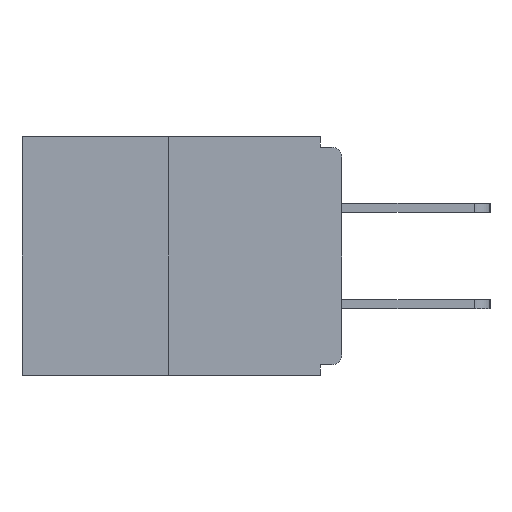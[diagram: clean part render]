
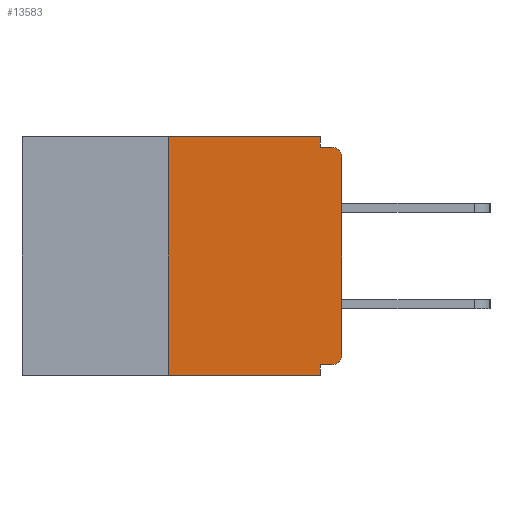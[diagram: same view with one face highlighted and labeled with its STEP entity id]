
A CAD part, left-side view. The second image highlights one B-rep face of the part: STEP entity #13583.
In plain terms, the highlighted planar face has unit normal (-1, 0, 0).
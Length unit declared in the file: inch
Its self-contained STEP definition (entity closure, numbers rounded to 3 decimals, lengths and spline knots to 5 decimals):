
#109 = CARTESIAN_POINT ( 'NONE',  ( 0., 0.031, -0.343 ) ) ;
#119 = ORIENTED_EDGE ( 'NONE', *, *, #7556, .F. ) ;
#203 = VECTOR ( 'NONE', #896, 39.37008 ) ;
#543 = DIRECTION ( 'NONE',  ( 0., -1., 0. ) ) ;
#877 = DIRECTION ( 'NONE',  ( 0., 0., 1. ) ) ;
#896 = DIRECTION ( 'NONE',  ( 0., -1., 0. ) ) ;
#913 = VERTEX_POINT ( 'NONE', #11214 ) ;
#1031 = FACE_OUTER_BOUND ( 'NONE', #7024, .T. ) ;
#1077 = VERTEX_POINT ( 'NONE', #8157 ) ;
#1084 = LINE ( 'NONE', #14793, #8114 ) ;
#1231 = CARTESIAN_POINT ( 'NONE',  ( 0., 0.031, -0.328 ) ) ;
#1260 = VERTEX_POINT ( 'NONE', #14646 ) ;
#1440 = EDGE_CURVE ( 'NONE', #9782, #913, #1084, .T. ) ;
#2194 = EDGE_CURVE ( 'NONE', #5644, #6878, #12732, .T. ) ;
#2239 = CARTESIAN_POINT ( 'NONE',  ( 0., 0.46, 0. ) ) ;
#2251 = ORIENTED_EDGE ( 'NONE', *, *, #5834, .T. ) ;
#2365 = VECTOR ( 'NONE', #12906, 39.37008 ) ;
#2741 = CARTESIAN_POINT ( 'NONE',  ( 0., 0.25, 0. ) ) ;
#2945 = VERTEX_POINT ( 'NONE', #2741 ) ;
#2973 = DIRECTION ( 'NONE',  ( 0., 0., 1. ) ) ;
#3752 = VERTEX_POINT ( 'NONE', #109 ) ;
#3786 = EDGE_CURVE ( 'NONE', #1260, #8052, #11182, .T. ) ;
#3901 = CARTESIAN_POINT ( 'NONE',  ( 0., 0.031, 0. ) ) ;
#3921 = ORIENTED_EDGE ( 'NONE', *, *, #3786, .T. ) ;
#4230 = VECTOR ( 'NONE', #543, 39.37008 ) ;
#4291 = ORIENTED_EDGE ( 'NONE', *, *, #6235, .F. ) ;
#4320 = LINE ( 'NONE', #8643, #4230 ) ;
#4352 = DIRECTION ( 'NONE',  ( 0., 0., -1. ) ) ;
#4830 = ORIENTED_EDGE ( 'NONE', *, *, #2194, .F. ) ;
#4906 = DIRECTION ( 'NONE',  ( 0., 0., -1. ) ) ;
#5644 = VERTEX_POINT ( 'NONE', #11697 ) ;
#5726 = DIRECTION ( 'NONE',  ( 1., 0., 0. ) ) ;
#5761 = CIRCLE ( 'NONE', #14292, 0.015 ) ;
#5834 = EDGE_CURVE ( 'NONE', #6703, #3752, #4320, .T. ) ;
#6095 = DIRECTION ( 'NONE',  ( 0., -1., 0. ) ) ;
#6235 = EDGE_CURVE ( 'NONE', #6703, #2945, #11353, .T. ) ;
#6686 = AXIS2_PLACEMENT_3D ( 'NONE', #11919, #8271, #8411 ) ;
#6703 = VERTEX_POINT ( 'NONE', #11028 ) ;
#6878 = VERTEX_POINT ( 'NONE', #1231 ) ;
#7024 = EDGE_LOOP ( 'NONE', ( #119, #4291, #2251, #10274, #4830, #8607, #3921, #10538, #7695, #13359 ) ) ;
#7244 = VECTOR ( 'NONE', #2973, 39.37008 ) ;
#7411 = CIRCLE ( 'NONE', #6686, 0.015 ) ;
#7556 = EDGE_CURVE ( 'NONE', #2945, #9782, #11292, .T. ) ;
#7694 = CARTESIAN_POINT ( 'NONE',  ( 0., 0.25, 0. ) ) ;
#7695 = ORIENTED_EDGE ( 'NONE', *, *, #10956, .F. ) ;
#7779 = CARTESIAN_POINT ( 'NONE',  ( 0., 0., -0.03 ) ) ;
#7876 = EDGE_CURVE ( 'NONE', #5644, #1260, #5761, .T. ) ;
#8052 = VERTEX_POINT ( 'NONE', #7779 ) ;
#8114 = VECTOR ( 'NONE', #4352, 39.37008 ) ;
#8157 = CARTESIAN_POINT ( 'NONE',  ( 0., 0.015, -0.015 ) ) ;
#8271 = DIRECTION ( 'NONE',  ( -1., 0., 0. ) ) ;
#8321 = DIRECTION ( 'NONE',  ( -1., 0., 0. ) ) ;
#8411 = DIRECTION ( 'NONE',  ( 0., 0., -1. ) ) ;
#8475 = CARTESIAN_POINT ( 'NONE',  ( 0., 0.015, -0.313 ) ) ;
#8607 = ORIENTED_EDGE ( 'NONE', *, *, #7876, .T. ) ;
#8643 = CARTESIAN_POINT ( 'NONE',  ( 0., 0.46, -0.343 ) ) ;
#8660 = CARTESIAN_POINT ( 'NONE',  ( 0., 0., 0. ) ) ;
#9391 = CARTESIAN_POINT ( 'NONE',  ( 0., 0.031, -0.343 ) ) ;
#9750 = LINE ( 'NONE', #9391, #2365 ) ;
#9782 = VERTEX_POINT ( 'NONE', #3901 ) ;
#10013 = CARTESIAN_POINT ( 'NONE',  ( 0., 0.46, 0. ) ) ;
#10101 = VECTOR ( 'NONE', #6095, 39.37008 ) ;
#10274 = ORIENTED_EDGE ( 'NONE', *, *, #12100, .F. ) ;
#10538 = ORIENTED_EDGE ( 'NONE', *, *, #10548, .T. ) ;
#10548 = EDGE_CURVE ( 'NONE', #8052, #1077, #7411, .T. ) ;
#10956 = EDGE_CURVE ( 'NONE', #913, #1077, #14238, .T. ) ;
#11028 = CARTESIAN_POINT ( 'NONE',  ( 0., 0.25, -0.343 ) ) ;
#11182 = LINE ( 'NONE', #8660, #7244 ) ;
#11214 = CARTESIAN_POINT ( 'NONE',  ( 0., 0.031, -0.015 ) ) ;
#11246 = VECTOR ( 'NONE', #12594, 39.37008 ) ;
#11292 = LINE ( 'NONE', #10013, #203 ) ;
#11353 = LINE ( 'NONE', #7694, #14169 ) ;
#11697 = CARTESIAN_POINT ( 'NONE',  ( 0., 0.015, -0.328 ) ) ;
#11919 = CARTESIAN_POINT ( 'NONE',  ( 0., 0.015, -0.03 ) ) ;
#12100 = EDGE_CURVE ( 'NONE', #6878, #3752, #9750, .T. ) ;
#12594 = DIRECTION ( 'NONE',  ( 0., 1., 0. ) ) ;
#12732 = LINE ( 'NONE', #14956, #11246 ) ;
#12906 = DIRECTION ( 'NONE',  ( 0., 0., -1. ) ) ;
#13359 = ORIENTED_EDGE ( 'NONE', *, *, #1440, .F. ) ;
#13583 = ADVANCED_FACE ( 'NONE', ( #1031 ), #13961, .F. ) ;
#13961 = PLANE ( 'NONE',  #14521 ) ;
#14169 = VECTOR ( 'NONE', #877, 39.37008 ) ;
#14170 = CARTESIAN_POINT ( 'NONE',  ( 0., 0., -0.015 ) ) ;
#14238 = LINE ( 'NONE', #14170, #10101 ) ;
#14292 = AXIS2_PLACEMENT_3D ( 'NONE', #8475, #8321, #4906 ) ;
#14521 = AXIS2_PLACEMENT_3D ( 'NONE', #2239, #5726, #15034 ) ;
#14646 = CARTESIAN_POINT ( 'NONE',  ( 0., 0., -0.313 ) ) ;
#14793 = CARTESIAN_POINT ( 'NONE',  ( 0., 0.031, 0. ) ) ;
#14956 = CARTESIAN_POINT ( 'NONE',  ( 0., 0., -0.328 ) ) ;
#15034 = DIRECTION ( 'NONE',  ( 0., 0., -1. ) ) ;
